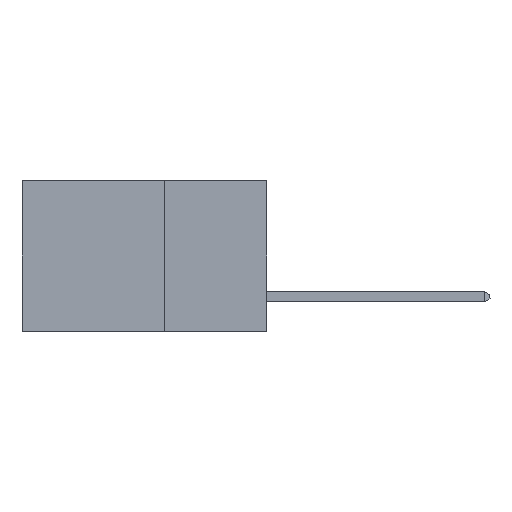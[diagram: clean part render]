
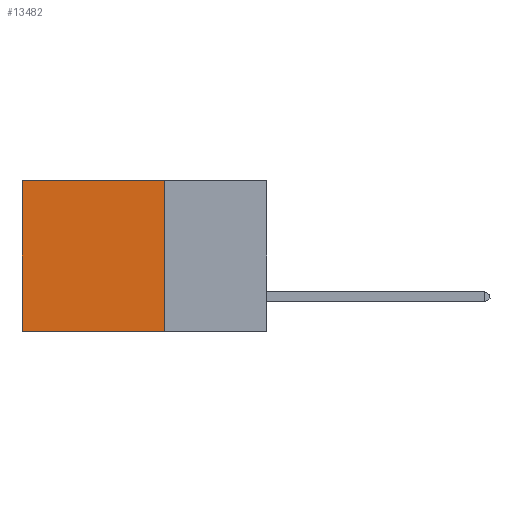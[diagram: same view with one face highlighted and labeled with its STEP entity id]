
A CAD part, left-side view. The second image highlights one B-rep face of the part: STEP entity #13482.
In plain terms, the highlighted planar face has unit normal (-1, 0, 0).
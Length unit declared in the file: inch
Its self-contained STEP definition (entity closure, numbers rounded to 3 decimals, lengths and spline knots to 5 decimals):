
#130 = VERTEX_POINT ( 'NONE', #1816 ) ;
#328 = CARTESIAN_POINT ( 'NONE',  ( 0.2875, 0.25, -0.37 ) ) ;
#349 = VECTOR ( 'NONE', #12836, 39.37008 ) ;
#1327 = PLANE ( 'NONE',  #20774 ) ;
#1816 = CARTESIAN_POINT ( 'NONE',  ( 0.2875, 0.6, -0.37 ) ) ;
#2000 = VECTOR ( 'NONE', #21788, 39.37008 ) ;
#3121 = EDGE_CURVE ( 'NONE', #8466, #4655, #17333, .T. ) ;
#3153 = CARTESIAN_POINT ( 'NONE',  ( 0.2875, 0.25, 0. ) ) ;
#4655 = VERTEX_POINT ( 'NONE', #5418 ) ;
#5418 = CARTESIAN_POINT ( 'NONE',  ( 0.2875, 0.6, 0. ) ) ;
#5571 = ORIENTED_EDGE ( 'NONE', *, *, #3121, .T. ) ;
#6829 = VECTOR ( 'NONE', #23306, 39.37008 ) ;
#7045 = VECTOR ( 'NONE', #20970, 39.37008 ) ;
#8466 = VERTEX_POINT ( 'NONE', #14005 ) ;
#9825 = CARTESIAN_POINT ( 'NONE',  ( 0.2875, 0.6, 0. ) ) ;
#10451 = EDGE_CURVE ( 'NONE', #8466, #23827, #20681, .T. ) ;
#10748 = DIRECTION ( 'NONE',  ( 1., 0., 0. ) ) ;
#10949 = CARTESIAN_POINT ( 'NONE',  ( 0.2875, 0.25, -0.37 ) ) ;
#11869 = EDGE_CURVE ( 'NONE', #4655, #130, #12605, .T. ) ;
#12605 = LINE ( 'NONE', #9825, #7045 ) ;
#12836 = DIRECTION ( 'NONE',  ( 0., 1., 0. ) ) ;
#13482 = ADVANCED_FACE ( 'NONE', ( #15420 ), #1327, .F. ) ;
#14005 = CARTESIAN_POINT ( 'NONE',  ( 0.2875, 0.25, 0. ) ) ;
#15420 = FACE_OUTER_BOUND ( 'NONE', #23557, .T. ) ;
#16743 = ORIENTED_EDGE ( 'NONE', *, *, #10451, .F. ) ;
#17333 = LINE ( 'NONE', #19494, #6829 ) ;
#19494 = CARTESIAN_POINT ( 'NONE',  ( 0.2875, 0.25, 0. ) ) ;
#20214 = LINE ( 'NONE', #10949, #349 ) ;
#20681 = LINE ( 'NONE', #3153, #2000 ) ;
#20774 = AXIS2_PLACEMENT_3D ( 'NONE', #21876, #10748, #23748 ) ;
#20970 = DIRECTION ( 'NONE',  ( 0., 0., -1. ) ) ;
#21018 = ORIENTED_EDGE ( 'NONE', *, *, #22093, .F. ) ;
#21788 = DIRECTION ( 'NONE',  ( 0., 0., -1. ) ) ;
#21876 = CARTESIAN_POINT ( 'NONE',  ( 0.2875, 0.25, 0. ) ) ;
#22093 = EDGE_CURVE ( 'NONE', #23827, #130, #20214, .T. ) ;
#22109 = ORIENTED_EDGE ( 'NONE', *, *, #11869, .T. ) ;
#23306 = DIRECTION ( 'NONE',  ( 0., 1., 0. ) ) ;
#23557 = EDGE_LOOP ( 'NONE', ( #22109, #21018, #16743, #5571 ) ) ;
#23748 = DIRECTION ( 'NONE',  ( 0., 0., -1. ) ) ;
#23827 = VERTEX_POINT ( 'NONE', #328 ) ;
